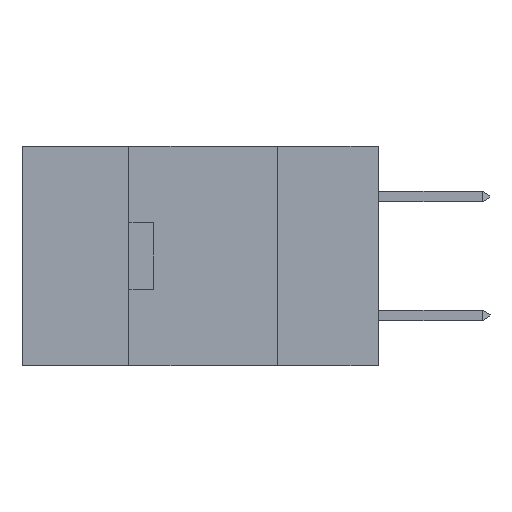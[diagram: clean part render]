
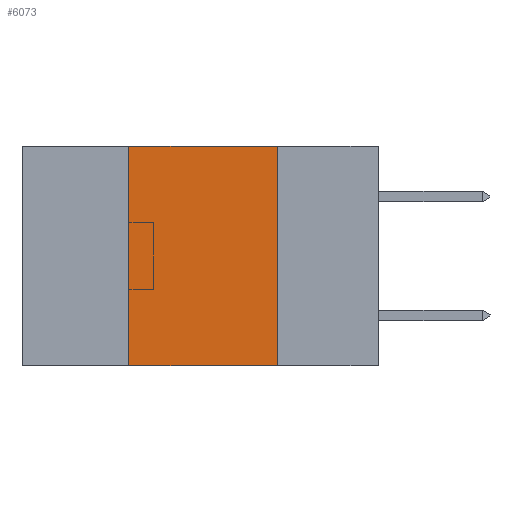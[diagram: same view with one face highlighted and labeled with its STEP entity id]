
A CAD part, left-side view. The second image highlights one B-rep face of the part: STEP entity #6073.
In plain terms, the highlighted planar face has unit normal (-1, 0, 0).
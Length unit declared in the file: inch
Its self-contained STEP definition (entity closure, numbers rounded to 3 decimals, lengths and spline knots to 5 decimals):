
#709 = DIRECTION ( 'NONE',  ( 0., 0., -1. ) ) ;
#3350 = ORIENTED_EDGE ( 'NONE', *, *, #21578, .F. ) ;
#4083 = DIRECTION ( 'NONE',  ( 0., -1., 0. ) ) ;
#4572 = EDGE_CURVE ( 'NONE', #7814, #10253, #24810, .T. ) ;
#6073 = ADVANCED_FACE ( 'NONE', ( #15137 ), #12133, .F. ) ;
#6237 = ORIENTED_EDGE ( 'NONE', *, *, #4572, .F. ) ;
#7560 = CARTESIAN_POINT ( 'NONE',  ( 0., 0.6, 0. ) ) ;
#7814 = VERTEX_POINT ( 'NONE', #13216 ) ;
#7875 = DIRECTION ( 'NONE',  ( 0., -1., 0. ) ) ;
#8742 = AXIS2_PLACEMENT_3D ( 'NONE', #7560, #14382, #709 ) ;
#9572 = VECTOR ( 'NONE', #7875, 39.37008 ) ;
#10253 = VERTEX_POINT ( 'NONE', #26361 ) ;
#10317 = VECTOR ( 'NONE', #16661, 39.37008 ) ;
#12133 = PLANE ( 'NONE',  #8742 ) ;
#12942 = VERTEX_POINT ( 'NONE', #21454 ) ;
#13216 = CARTESIAN_POINT ( 'NONE',  ( 0., 0.42, -0.37 ) ) ;
#13481 = DIRECTION ( 'NONE',  ( 0., 0., 1. ) ) ;
#14382 = DIRECTION ( 'NONE',  ( 1., 0., 0. ) ) ;
#14784 = VERTEX_POINT ( 'NONE', #25397 ) ;
#15137 = FACE_OUTER_BOUND ( 'NONE', #16933, .T. ) ;
#15553 = LINE ( 'NONE', #27774, #9572 ) ;
#15947 = EDGE_CURVE ( 'NONE', #7814, #14784, #15553, .T. ) ;
#16284 = LINE ( 'NONE', #23245, #10317 ) ;
#16661 = DIRECTION ( 'NONE',  ( 0., 0., -1. ) ) ;
#16933 = EDGE_LOOP ( 'NONE', ( #3350, #22043, #6237, #24798 ) ) ;
#19775 = CARTESIAN_POINT ( 'NONE',  ( 0., 0.6, 0. ) ) ;
#20091 = CARTESIAN_POINT ( 'NONE',  ( 0., 0.42, -0.37 ) ) ;
#20826 = VECTOR ( 'NONE', #4083, 39.37008 ) ;
#21187 = EDGE_CURVE ( 'NONE', #10253, #12942, #26651, .T. ) ;
#21454 = CARTESIAN_POINT ( 'NONE',  ( 0., 0.17, 0. ) ) ;
#21578 = EDGE_CURVE ( 'NONE', #12942, #14784, #16284, .T. ) ;
#22043 = ORIENTED_EDGE ( 'NONE', *, *, #21187, .F. ) ;
#23245 = CARTESIAN_POINT ( 'NONE',  ( 0., 0.17, -0.37 ) ) ;
#24120 = VECTOR ( 'NONE', #13481, 39.37008 ) ;
#24798 = ORIENTED_EDGE ( 'NONE', *, *, #15947, .T. ) ;
#24810 = LINE ( 'NONE', #20091, #24120 ) ;
#25397 = CARTESIAN_POINT ( 'NONE',  ( 0., 0.17, -0.37 ) ) ;
#26361 = CARTESIAN_POINT ( 'NONE',  ( 0., 0.42, 0. ) ) ;
#26651 = LINE ( 'NONE', #19775, #20826 ) ;
#27774 = CARTESIAN_POINT ( 'NONE',  ( 0., 0.6, -0.37 ) ) ;
